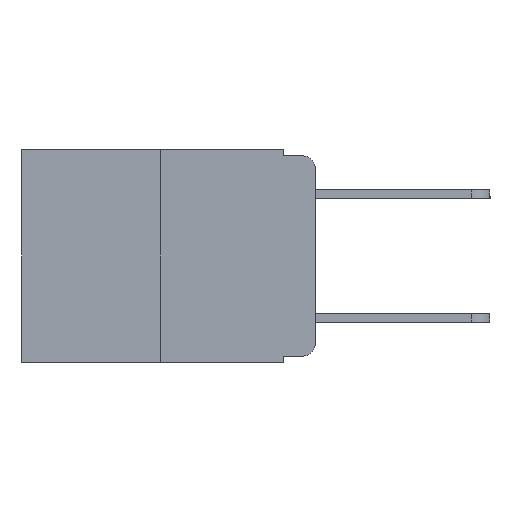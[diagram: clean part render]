
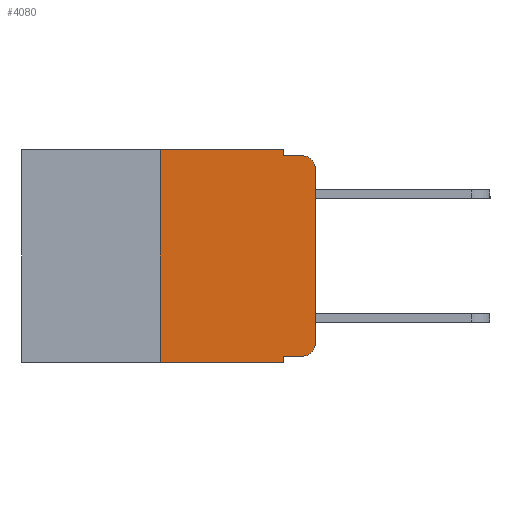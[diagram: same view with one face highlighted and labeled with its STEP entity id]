
A CAD part, left-side view. The second image highlights one B-rep face of the part: STEP entity #4080.
In plain terms, the highlighted planar face has unit normal (-1, 0, 0).
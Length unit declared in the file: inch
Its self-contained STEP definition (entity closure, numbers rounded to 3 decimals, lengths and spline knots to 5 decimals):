
#57 = VERTEX_POINT ( 'NONE', #14239 ) ;
#253 = EDGE_CURVE ( 'NONE', #4330, #2754, #9841, .T. ) ;
#273 = CARTESIAN_POINT ( 'NONE',  ( 0., 0.051, -0.01 ) ) ;
#946 = EDGE_CURVE ( 'NONE', #4148, #2859, #6962, .T. ) ;
#1058 = LINE ( 'NONE', #16484, #8458 ) ;
#1866 = VECTOR ( 'NONE', #13217, 39.37008 ) ;
#2754 = VERTEX_POINT ( 'NONE', #17249 ) ;
#2774 = DIRECTION ( 'NONE',  ( 0., 0., -1. ) ) ;
#2811 = VECTOR ( 'NONE', #2774, 39.37008 ) ;
#2859 = VERTEX_POINT ( 'NONE', #12381 ) ;
#3123 = DIRECTION ( 'NONE',  ( 0., 0., 1. ) ) ;
#3495 = VERTEX_POINT ( 'NONE', #13678 ) ;
#3539 = VECTOR ( 'NONE', #9045, 39.37008 ) ;
#3752 = CARTESIAN_POINT ( 'NONE',  ( 0., 0.02, -0.333 ) ) ;
#3783 = CIRCLE ( 'NONE', #11198, 0.02 ) ;
#3837 = VECTOR ( 'NONE', #13869, 39.37008 ) ;
#3982 = CARTESIAN_POINT ( 'NONE',  ( 0., 0.051, 0. ) ) ;
#4080 = ADVANCED_FACE ( 'NONE', ( #12752 ), #15302, .F. ) ;
#4148 = VERTEX_POINT ( 'NONE', #9101 ) ;
#4196 = ORIENTED_EDGE ( 'NONE', *, *, #11703, .T. ) ;
#4330 = VERTEX_POINT ( 'NONE', #17688 ) ;
#4764 = AXIS2_PLACEMENT_3D ( 'NONE', #10013, #10032, #9937 ) ;
#5276 = VECTOR ( 'NONE', #3123, 39.37008 ) ;
#5370 = ORIENTED_EDGE ( 'NONE', *, *, #16509, .T. ) ;
#5554 = DIRECTION ( 'NONE',  ( -1., 0., 0. ) ) ;
#5806 = ORIENTED_EDGE ( 'NONE', *, *, #17244, .T. ) ;
#6139 = VERTEX_POINT ( 'NONE', #12363 ) ;
#6163 = CARTESIAN_POINT ( 'NONE',  ( 0., 0., 0. ) ) ;
#6278 = ORIENTED_EDGE ( 'NONE', *, *, #946, .F. ) ;
#6406 = CARTESIAN_POINT ( 'NONE',  ( 0., 0.473, 0. ) ) ;
#6463 = ORIENTED_EDGE ( 'NONE', *, *, #15001, .F. ) ;
#6680 = ORIENTED_EDGE ( 'NONE', *, *, #253, .T. ) ;
#6810 = DIRECTION ( 'NONE',  ( 0., -1., 0. ) ) ;
#6897 = LINE ( 'NONE', #3982, #2811 ) ;
#6962 = LINE ( 'NONE', #6406, #16639 ) ;
#6992 = CARTESIAN_POINT ( 'NONE',  ( 0., 0.473, -0.343 ) ) ;
#7003 = ORIENTED_EDGE ( 'NONE', *, *, #14194, .F. ) ;
#7683 = CARTESIAN_POINT ( 'NONE',  ( 0., 0.051, -0.333 ) ) ;
#7842 = LINE ( 'NONE', #10057, #3837 ) ;
#8458 = VECTOR ( 'NONE', #17600, 39.37008 ) ;
#8486 = LINE ( 'NONE', #7683, #3539 ) ;
#8862 = AXIS2_PLACEMENT_3D ( 'NONE', #13621, #5554, #14806 ) ;
#8947 = CARTESIAN_POINT ( 'NONE',  ( 0., 0.02, -0.313 ) ) ;
#9045 = DIRECTION ( 'NONE',  ( 0., -1., 0. ) ) ;
#9101 = CARTESIAN_POINT ( 'NONE',  ( 0., 0.25, 0. ) ) ;
#9296 = ORIENTED_EDGE ( 'NONE', *, *, #12552, .T. ) ;
#9318 = ORIENTED_EDGE ( 'NONE', *, *, #15758, .F. ) ;
#9841 = LINE ( 'NONE', #6992, #1866 ) ;
#9937 = DIRECTION ( 'NONE',  ( 0., 0., -1. ) ) ;
#10013 = CARTESIAN_POINT ( 'NONE',  ( 0., 0.473, 0. ) ) ;
#10032 = DIRECTION ( 'NONE',  ( 1., 0., 0. ) ) ;
#10057 = CARTESIAN_POINT ( 'NONE',  ( 0., 0.25, 0. ) ) ;
#10254 = DIRECTION ( 'NONE',  ( 0., 0., -1. ) ) ;
#10628 = VERTEX_POINT ( 'NONE', #13289 ) ;
#10726 = CIRCLE ( 'NONE', #8862, 0.02 ) ;
#11198 = AXIS2_PLACEMENT_3D ( 'NONE', #8947, #17417, #10254 ) ;
#11316 = ORIENTED_EDGE ( 'NONE', *, *, #13419, .F. ) ;
#11326 = VECTOR ( 'NONE', #6810, 39.37008 ) ;
#11703 = EDGE_CURVE ( 'NONE', #15745, #6139, #3783, .T. ) ;
#11768 = CARTESIAN_POINT ( 'NONE',  ( 0., 0.051, -0.01 ) ) ;
#12130 = LINE ( 'NONE', #6163, #5276 ) ;
#12363 = CARTESIAN_POINT ( 'NONE',  ( 0., 0., -0.313 ) ) ;
#12381 = CARTESIAN_POINT ( 'NONE',  ( 0., 0.051, 0. ) ) ;
#12552 = EDGE_CURVE ( 'NONE', #3495, #15745, #8486, .T. ) ;
#12695 = EDGE_LOOP ( 'NONE', ( #5370, #5806, #9318, #6463, #6278, #7003, #6680, #11316, #9296, #4196 ) ) ;
#12752 = FACE_OUTER_BOUND ( 'NONE', #12695, .T. ) ;
#13217 = DIRECTION ( 'NONE',  ( 0., -1., 0. ) ) ;
#13289 = CARTESIAN_POINT ( 'NONE',  ( 0., 0., -0.03 ) ) ;
#13419 = EDGE_CURVE ( 'NONE', #3495, #2754, #1058, .T. ) ;
#13621 = CARTESIAN_POINT ( 'NONE',  ( 0., 0.02, -0.03 ) ) ;
#13678 = CARTESIAN_POINT ( 'NONE',  ( 0., 0.051, -0.333 ) ) ;
#13869 = DIRECTION ( 'NONE',  ( 0., 0., 1. ) ) ;
#14194 = EDGE_CURVE ( 'NONE', #4330, #4148, #7842, .T. ) ;
#14239 = CARTESIAN_POINT ( 'NONE',  ( 0., 0.02, -0.01 ) ) ;
#14523 = VERTEX_POINT ( 'NONE', #11768 ) ;
#14629 = LINE ( 'NONE', #273, #11326 ) ;
#14768 = DIRECTION ( 'NONE',  ( 0., -1., 0. ) ) ;
#14806 = DIRECTION ( 'NONE',  ( 0., 0., -1. ) ) ;
#15001 = EDGE_CURVE ( 'NONE', #2859, #14523, #6897, .T. ) ;
#15302 = PLANE ( 'NONE',  #4764 ) ;
#15745 = VERTEX_POINT ( 'NONE', #3752 ) ;
#15758 = EDGE_CURVE ( 'NONE', #14523, #57, #14629, .T. ) ;
#16484 = CARTESIAN_POINT ( 'NONE',  ( 0., 0.051, 0. ) ) ;
#16509 = EDGE_CURVE ( 'NONE', #6139, #10628, #12130, .T. ) ;
#16639 = VECTOR ( 'NONE', #14768, 39.37008 ) ;
#17244 = EDGE_CURVE ( 'NONE', #10628, #57, #10726, .T. ) ;
#17249 = CARTESIAN_POINT ( 'NONE',  ( 0., 0.051, -0.343 ) ) ;
#17417 = DIRECTION ( 'NONE',  ( -1., 0., 0. ) ) ;
#17600 = DIRECTION ( 'NONE',  ( 0., 0., -1. ) ) ;
#17688 = CARTESIAN_POINT ( 'NONE',  ( 0., 0.25, -0.343 ) ) ;
